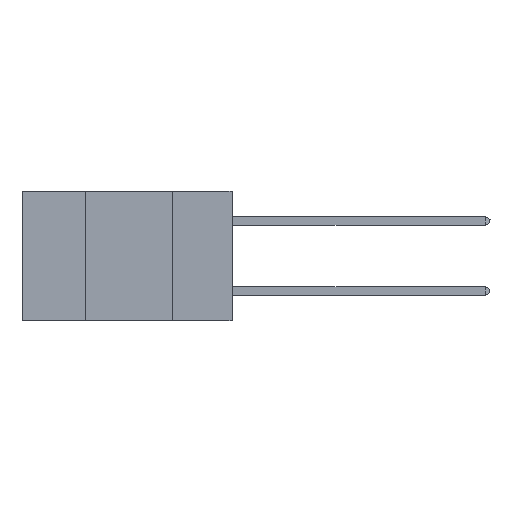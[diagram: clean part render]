
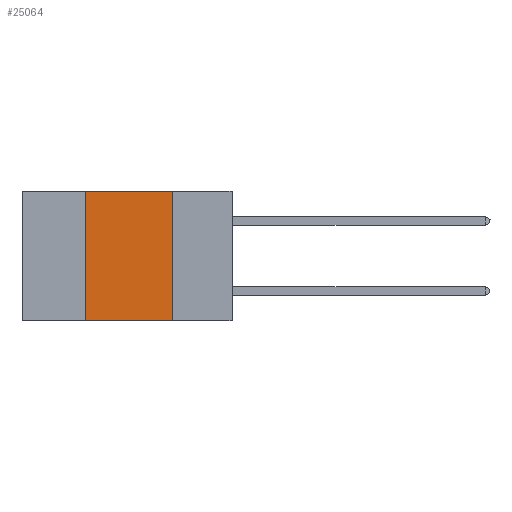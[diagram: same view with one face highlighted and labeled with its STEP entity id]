
A CAD part, left-side view. The second image highlights one B-rep face of the part: STEP entity #25064.
In plain terms, the highlighted planar face has unit normal (-1, 0, 0).
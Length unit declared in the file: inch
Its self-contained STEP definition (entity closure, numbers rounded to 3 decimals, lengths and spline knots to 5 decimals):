
#46 = CARTESIAN_POINT ( 'NONE',  ( 0., 0.6, 0. ) ) ;
#2120 = CARTESIAN_POINT ( 'NONE',  ( 0., 0.6, 0. ) ) ;
#3068 = CARTESIAN_POINT ( 'NONE',  ( 0., 0.42, 0. ) ) ;
#3614 = VERTEX_POINT ( 'NONE', #10958 ) ;
#4449 = CARTESIAN_POINT ( 'NONE',  ( 0., 0.6, -0.37 ) ) ;
#4880 = EDGE_CURVE ( 'NONE', #3614, #26316, #4970, .T. ) ;
#4970 = LINE ( 'NONE', #12760, #31632 ) ;
#5124 = LINE ( 'NONE', #46, #31544 ) ;
#7049 = CARTESIAN_POINT ( 'NONE',  ( 0., 0.17, -0.37 ) ) ;
#7673 = DIRECTION ( 'NONE',  ( 0., -1., 0. ) ) ;
#9635 = EDGE_CURVE ( 'NONE', #25480, #31792, #13569, .T. ) ;
#10392 = DIRECTION ( 'NONE',  ( 0., -1., 0. ) ) ;
#10958 = CARTESIAN_POINT ( 'NONE',  ( 0., 0.17, 0. ) ) ;
#11704 = EDGE_LOOP ( 'NONE', ( #19223, #31182, #29830, #32856 ) ) ;
#12622 = DIRECTION ( 'NONE',  ( 1., 0., 0. ) ) ;
#12760 = CARTESIAN_POINT ( 'NONE',  ( 0., 0.17, 0. ) ) ;
#13569 = LINE ( 'NONE', #3068, #19497 ) ;
#14161 = EDGE_CURVE ( 'NONE', #31792, #3614, #5124, .T. ) ;
#15321 = FACE_OUTER_BOUND ( 'NONE', #11704, .T. ) ;
#17281 = VECTOR ( 'NONE', #7673, 39.37008 ) ;
#17924 = EDGE_CURVE ( 'NONE', #25480, #26316, #30764, .T. ) ;
#18799 = DIRECTION ( 'NONE',  ( 0., 0., 1. ) ) ;
#19223 = ORIENTED_EDGE ( 'NONE', *, *, #4880, .F. ) ;
#19497 = VECTOR ( 'NONE', #18799, 39.37008 ) ;
#20218 = PLANE ( 'NONE',  #23616 ) ;
#20853 = CARTESIAN_POINT ( 'NONE',  ( 0., 0.42, 0. ) ) ;
#22407 = DIRECTION ( 'NONE',  ( 0., 0., -1. ) ) ;
#23616 = AXIS2_PLACEMENT_3D ( 'NONE', #2120, #12622, #22407 ) ;
#25052 = DIRECTION ( 'NONE',  ( 0., 0., -1. ) ) ;
#25064 = ADVANCED_FACE ( 'NONE', ( #15321 ), #20218, .F. ) ;
#25480 = VERTEX_POINT ( 'NONE', #33124 ) ;
#26316 = VERTEX_POINT ( 'NONE', #7049 ) ;
#29830 = ORIENTED_EDGE ( 'NONE', *, *, #9635, .F. ) ;
#30764 = LINE ( 'NONE', #4449, #17281 ) ;
#31182 = ORIENTED_EDGE ( 'NONE', *, *, #14161, .F. ) ;
#31544 = VECTOR ( 'NONE', #10392, 39.37008 ) ;
#31632 = VECTOR ( 'NONE', #25052, 39.37008 ) ;
#31792 = VERTEX_POINT ( 'NONE', #20853 ) ;
#32856 = ORIENTED_EDGE ( 'NONE', *, *, #17924, .T. ) ;
#33124 = CARTESIAN_POINT ( 'NONE',  ( 0., 0.42, -0.37 ) ) ;
